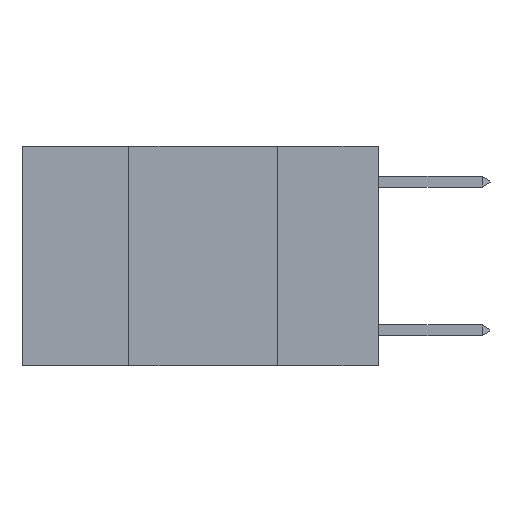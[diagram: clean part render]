
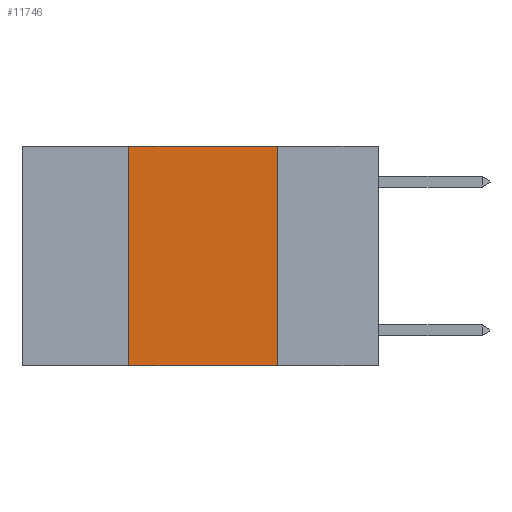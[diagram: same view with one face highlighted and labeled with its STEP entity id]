
A CAD part, left-side view. The second image highlights one B-rep face of the part: STEP entity #11746.
In plain terms, the highlighted planar face has unit normal (-1, 0, 0).
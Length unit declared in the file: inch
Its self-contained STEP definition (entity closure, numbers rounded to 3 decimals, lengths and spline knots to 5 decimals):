
#122 = LINE ( 'NONE', #11912, #10822 ) ;
#908 = DIRECTION ( 'NONE',  ( 0., -1., 0. ) ) ;
#987 = CARTESIAN_POINT ( 'NONE',  ( 0., 0.17, 0. ) ) ;
#3741 = DIRECTION ( 'NONE',  ( 0., 0., -1. ) ) ;
#3961 = DIRECTION ( 'NONE',  ( 0., 0., -1. ) ) ;
#4584 = LINE ( 'NONE', #5556, #7000 ) ;
#4777 = VERTEX_POINT ( 'NONE', #9647 ) ;
#5525 = LINE ( 'NONE', #987, #8836 ) ;
#5543 = EDGE_CURVE ( 'NONE', #4777, #12685, #4584, .T. ) ;
#5556 = CARTESIAN_POINT ( 'NONE',  ( 0., 0.6, 0. ) ) ;
#6906 = AXIS2_PLACEMENT_3D ( 'NONE', #10953, #12329, #3961 ) ;
#7000 = VECTOR ( 'NONE', #16793, 39.37008 ) ;
#7401 = ORIENTED_EDGE ( 'NONE', *, *, #5543, .F. ) ;
#7874 = CARTESIAN_POINT ( 'NONE',  ( 0., 0.42, -0.37 ) ) ;
#8045 = LINE ( 'NONE', #17545, #15019 ) ;
#8465 = ORIENTED_EDGE ( 'NONE', *, *, #15831, .F. ) ;
#8816 = CARTESIAN_POINT ( 'NONE',  ( 0., 0.17, -0.37 ) ) ;
#8836 = VECTOR ( 'NONE', #3741, 39.37008 ) ;
#9540 = PLANE ( 'NONE',  #6906 ) ;
#9647 = CARTESIAN_POINT ( 'NONE',  ( 0., 0.42, 0. ) ) ;
#9764 = VERTEX_POINT ( 'NONE', #7874 ) ;
#10822 = VECTOR ( 'NONE', #14720, 39.37008 ) ;
#10953 = CARTESIAN_POINT ( 'NONE',  ( 0., 0.6, 0. ) ) ;
#11746 = ADVANCED_FACE ( 'NONE', ( #15806 ), #9540, .F. ) ;
#11912 = CARTESIAN_POINT ( 'NONE',  ( 0., 0.42, 0. ) ) ;
#11920 = ORIENTED_EDGE ( 'NONE', *, *, #14901, .F. ) ;
#12329 = DIRECTION ( 'NONE',  ( 1., 0., 0. ) ) ;
#12608 = ORIENTED_EDGE ( 'NONE', *, *, #13013, .T. ) ;
#12685 = VERTEX_POINT ( 'NONE', #12709 ) ;
#12709 = CARTESIAN_POINT ( 'NONE',  ( 0., 0.17, 0. ) ) ;
#13013 = EDGE_CURVE ( 'NONE', #9764, #16136, #8045, .T. ) ;
#13765 = EDGE_LOOP ( 'NONE', ( #8465, #7401, #11920, #12608 ) ) ;
#14720 = DIRECTION ( 'NONE',  ( 0., 0., 1. ) ) ;
#14901 = EDGE_CURVE ( 'NONE', #9764, #4777, #122, .T. ) ;
#15019 = VECTOR ( 'NONE', #908, 39.37008 ) ;
#15806 = FACE_OUTER_BOUND ( 'NONE', #13765, .T. ) ;
#15831 = EDGE_CURVE ( 'NONE', #12685, #16136, #5525, .T. ) ;
#16136 = VERTEX_POINT ( 'NONE', #8816 ) ;
#16793 = DIRECTION ( 'NONE',  ( 0., -1., 0. ) ) ;
#17545 = CARTESIAN_POINT ( 'NONE',  ( 0., 0.6, -0.37 ) ) ;
